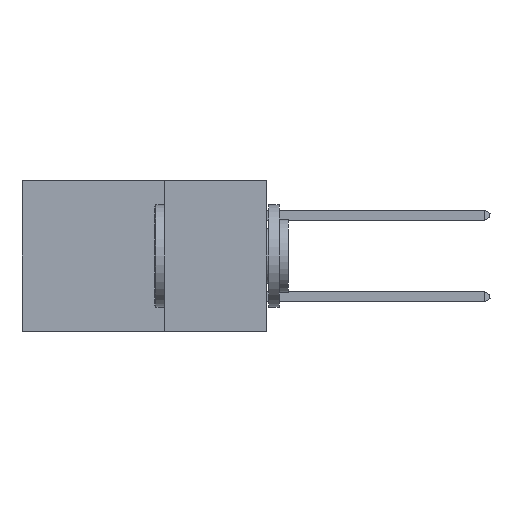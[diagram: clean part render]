
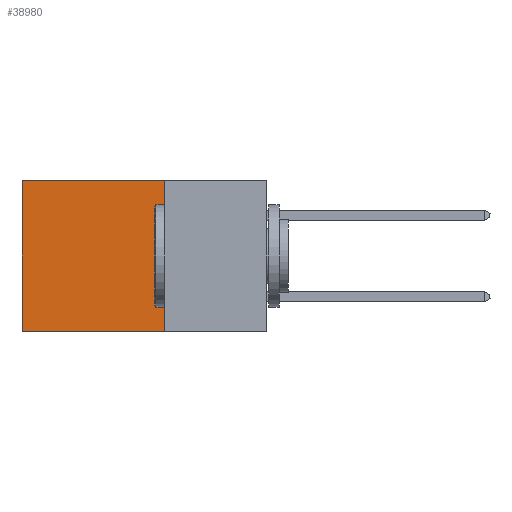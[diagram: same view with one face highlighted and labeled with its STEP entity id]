
A CAD part, left-side view. The second image highlights one B-rep face of the part: STEP entity #38980.
In plain terms, the highlighted planar face has unit normal (-1, 0, 0).
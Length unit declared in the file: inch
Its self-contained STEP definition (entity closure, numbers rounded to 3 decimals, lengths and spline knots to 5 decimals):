
#264 = CARTESIAN_POINT ( 'NONE',  ( 0.2875, 0.25, -0.37 ) ) ;
#1150 = DIRECTION ( 'NONE',  ( 0., 1., 0. ) ) ;
#2856 = VECTOR ( 'NONE', #9141, 39.37008 ) ;
#3946 = CARTESIAN_POINT ( 'NONE',  ( 0.2875, 0.25, -0.37 ) ) ;
#4414 = ORIENTED_EDGE ( 'NONE', *, *, #43566, .F. ) ;
#6162 = VECTOR ( 'NONE', #37808, 39.37008 ) ;
#6542 = EDGE_CURVE ( 'NONE', #16220, #38756, #11728, .T. ) ;
#9141 = DIRECTION ( 'NONE',  ( 0., 0., -1. ) ) ;
#9179 = DIRECTION ( 'NONE',  ( 0., 0., -1. ) ) ;
#9713 = VECTOR ( 'NONE', #1150, 39.37008 ) ;
#11728 = LINE ( 'NONE', #12705, #2856 ) ;
#12705 = CARTESIAN_POINT ( 'NONE',  ( 0.2875, 0.6, 0. ) ) ;
#13621 = CARTESIAN_POINT ( 'NONE',  ( 0.2875, 0.25, 0. ) ) ;
#14800 = VERTEX_POINT ( 'NONE', #264 ) ;
#16220 = VERTEX_POINT ( 'NONE', #43934 ) ;
#18271 = ORIENTED_EDGE ( 'NONE', *, *, #23858, .F. ) ;
#19172 = CARTESIAN_POINT ( 'NONE',  ( 0.2875, 0.6, -0.37 ) ) ;
#19773 = CARTESIAN_POINT ( 'NONE',  ( 0.2875, 0.25, 0. ) ) ;
#20800 = DIRECTION ( 'NONE',  ( 0., 0., -1. ) ) ;
#23399 = CARTESIAN_POINT ( 'NONE',  ( 0.2875, 0.25, 0. ) ) ;
#23858 = EDGE_CURVE ( 'NONE', #31284, #14800, #39809, .T. ) ;
#25873 = LINE ( 'NONE', #3946, #9713 ) ;
#27452 = CARTESIAN_POINT ( 'NONE',  ( 0.2875, 0.25, 0. ) ) ;
#27825 = EDGE_CURVE ( 'NONE', #31284, #16220, #37846, .T. ) ;
#31284 = VERTEX_POINT ( 'NONE', #23399 ) ;
#34254 = ORIENTED_EDGE ( 'NONE', *, *, #6542, .T. ) ;
#37773 = PLANE ( 'NONE',  #40278 ) ;
#37808 = DIRECTION ( 'NONE',  ( 0., 1., 0. ) ) ;
#37846 = LINE ( 'NONE', #27452, #6162 ) ;
#38145 = VECTOR ( 'NONE', #20800, 39.37008 ) ;
#38756 = VERTEX_POINT ( 'NONE', #19172 ) ;
#38980 = ADVANCED_FACE ( 'NONE', ( #41320 ), #37773, .F. ) ;
#39809 = LINE ( 'NONE', #13621, #38145 ) ;
#40278 = AXIS2_PLACEMENT_3D ( 'NONE', #19773, #44549, #9179 ) ;
#41320 = FACE_OUTER_BOUND ( 'NONE', #44212, .T. ) ;
#43566 = EDGE_CURVE ( 'NONE', #14800, #38756, #25873, .T. ) ;
#43934 = CARTESIAN_POINT ( 'NONE',  ( 0.2875, 0.6, 0. ) ) ;
#44212 = EDGE_LOOP ( 'NONE', ( #34254, #4414, #18271, #45270 ) ) ;
#44549 = DIRECTION ( 'NONE',  ( 1., 0., 0. ) ) ;
#45270 = ORIENTED_EDGE ( 'NONE', *, *, #27825, .T. ) ;
